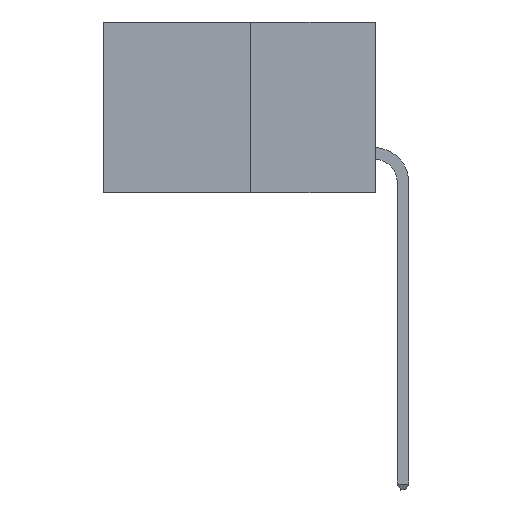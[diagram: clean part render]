
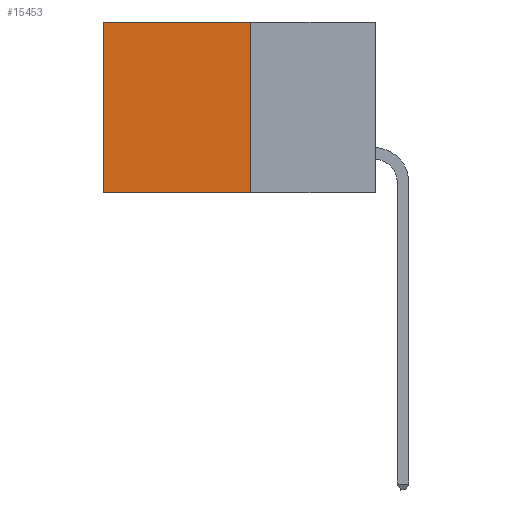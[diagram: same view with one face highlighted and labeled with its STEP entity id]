
A CAD part, left-side view. The second image highlights one B-rep face of the part: STEP entity #15453.
In plain terms, the highlighted planar face has unit normal (-1, 0, 0).
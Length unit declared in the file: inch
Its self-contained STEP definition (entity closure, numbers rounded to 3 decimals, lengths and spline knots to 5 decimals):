
#577 = EDGE_LOOP ( 'NONE', ( #2605, #13616, #22035, #15024 ) ) ;
#1151 = VERTEX_POINT ( 'NONE', #16110 ) ;
#1804 = CARTESIAN_POINT ( 'NONE',  ( 0.277, 0.59, 0. ) ) ;
#2103 = VECTOR ( 'NONE', #14090, 39.37008 ) ;
#2378 = CARTESIAN_POINT ( 'NONE',  ( 0.277, 0.27, -0.37 ) ) ;
#2419 = EDGE_CURVE ( 'NONE', #1151, #7960, #15029, .T. ) ;
#2605 = ORIENTED_EDGE ( 'NONE', *, *, #17317, .T. ) ;
#4013 = DIRECTION ( 'NONE',  ( 0., 0., -1. ) ) ;
#5281 = CARTESIAN_POINT ( 'NONE',  ( 0.277, 0.59, -0.37 ) ) ;
#7049 = LINE ( 'NONE', #2378, #20391 ) ;
#7942 = CARTESIAN_POINT ( 'NONE',  ( 0.277, 0.27, 0. ) ) ;
#7960 = VERTEX_POINT ( 'NONE', #1804 ) ;
#8723 = CARTESIAN_POINT ( 'NONE',  ( 0.277, 0.27, -0.37 ) ) ;
#9304 = PLANE ( 'NONE',  #12978 ) ;
#10019 = CARTESIAN_POINT ( 'NONE',  ( 0.277, 0.59, -0.37 ) ) ;
#10423 = LINE ( 'NONE', #5281, #15022 ) ;
#11474 = VERTEX_POINT ( 'NONE', #10019 ) ;
#12786 = CARTESIAN_POINT ( 'NONE',  ( 0.277, 0.27, -0.37 ) ) ;
#12957 = EDGE_CURVE ( 'NONE', #15050, #11474, #20043, .T. ) ;
#12978 = AXIS2_PLACEMENT_3D ( 'NONE', #12786, #14555, #4013 ) ;
#13616 = ORIENTED_EDGE ( 'NONE', *, *, #12957, .F. ) ;
#14072 = DIRECTION ( 'NONE',  ( 0., 0., -1. ) ) ;
#14090 = DIRECTION ( 'NONE',  ( 0., 1., 0. ) ) ;
#14555 = DIRECTION ( 'NONE',  ( 1., 0., 0. ) ) ;
#14865 = VECTOR ( 'NONE', #20804, 39.37008 ) ;
#15022 = VECTOR ( 'NONE', #14072, 39.37008 ) ;
#15024 = ORIENTED_EDGE ( 'NONE', *, *, #2419, .T. ) ;
#15029 = LINE ( 'NONE', #7942, #2103 ) ;
#15050 = VERTEX_POINT ( 'NONE', #18345 ) ;
#15124 = FACE_OUTER_BOUND ( 'NONE', #577, .T. ) ;
#15453 = ADVANCED_FACE ( 'NONE', ( #15124 ), #9304, .F. ) ;
#16110 = CARTESIAN_POINT ( 'NONE',  ( 0.277, 0.27, 0. ) ) ;
#17317 = EDGE_CURVE ( 'NONE', #7960, #11474, #10423, .T. ) ;
#18183 = DIRECTION ( 'NONE',  ( 0., 0., -1. ) ) ;
#18345 = CARTESIAN_POINT ( 'NONE',  ( 0.277, 0.27, -0.37 ) ) ;
#20043 = LINE ( 'NONE', #8723, #14865 ) ;
#20391 = VECTOR ( 'NONE', #18183, 39.37008 ) ;
#20804 = DIRECTION ( 'NONE',  ( 0., 1., 0. ) ) ;
#22035 = ORIENTED_EDGE ( 'NONE', *, *, #22576, .F. ) ;
#22576 = EDGE_CURVE ( 'NONE', #1151, #15050, #7049, .T. ) ;
